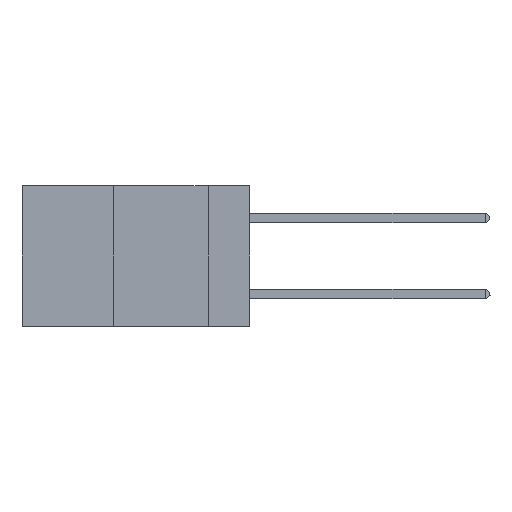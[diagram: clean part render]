
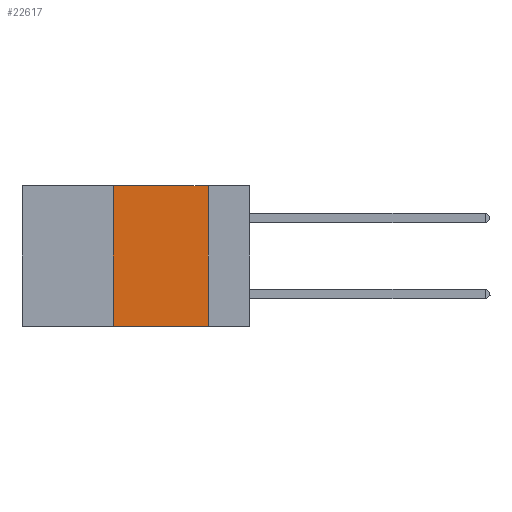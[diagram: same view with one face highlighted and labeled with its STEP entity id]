
A CAD part, left-side view. The second image highlights one B-rep face of the part: STEP entity #22617.
In plain terms, the highlighted planar face has unit normal (-1, 0, 0).
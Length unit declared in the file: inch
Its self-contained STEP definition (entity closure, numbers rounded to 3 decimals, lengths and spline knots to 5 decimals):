
#1865 = VERTEX_POINT ( 'NONE', #22115 ) ;
#2059 = CARTESIAN_POINT ( 'NONE',  ( 0., 0.11, 0. ) ) ;
#3013 = EDGE_LOOP ( 'NONE', ( #31427, #17094, #28552, #44495 ) ) ;
#3513 = DIRECTION ( 'NONE',  ( 0., 0., -1. ) ) ;
#3984 = CARTESIAN_POINT ( 'NONE',  ( 0., 0.11, 0. ) ) ;
#5112 = LINE ( 'NONE', #32090, #32329 ) ;
#7282 = DIRECTION ( 'NONE',  ( 0., -1., 0. ) ) ;
#7284 = CARTESIAN_POINT ( 'NONE',  ( 0., 0.6, 0. ) ) ;
#9518 = DIRECTION ( 'NONE',  ( 0., -1., 0. ) ) ;
#12068 = LINE ( 'NONE', #3984, #15471 ) ;
#12148 = EDGE_CURVE ( 'NONE', #43006, #32721, #12068, .T. ) ;
#15296 = FACE_OUTER_BOUND ( 'NONE', #3013, .T. ) ;
#15455 = CARTESIAN_POINT ( 'NONE',  ( 0., 0.11, -0.37 ) ) ;
#15471 = VECTOR ( 'NONE', #3513, 39.37008 ) ;
#17094 = ORIENTED_EDGE ( 'NONE', *, *, #31562, .F. ) ;
#21498 = PLANE ( 'NONE',  #27385 ) ;
#22115 = CARTESIAN_POINT ( 'NONE',  ( 0., 0.36, 0. ) ) ;
#22410 = CARTESIAN_POINT ( 'NONE',  ( 0., 0.36, -0.37 ) ) ;
#22533 = EDGE_CURVE ( 'NONE', #39396, #1865, #28602, .T. ) ;
#22617 = ADVANCED_FACE ( 'NONE', ( #15296 ), #21498, .F. ) ;
#24997 = EDGE_CURVE ( 'NONE', #39396, #32721, #5112, .T. ) ;
#27385 = AXIS2_PLACEMENT_3D ( 'NONE', #7284, #32092, #28964 ) ;
#28552 = ORIENTED_EDGE ( 'NONE', *, *, #22533, .F. ) ;
#28602 = LINE ( 'NONE', #39047, #42508 ) ;
#28964 = DIRECTION ( 'NONE',  ( 0., 0., -1. ) ) ;
#29127 = VECTOR ( 'NONE', #9518, 39.37008 ) ;
#31427 = ORIENTED_EDGE ( 'NONE', *, *, #12148, .F. ) ;
#31562 = EDGE_CURVE ( 'NONE', #1865, #43006, #38551, .T. ) ;
#32090 = CARTESIAN_POINT ( 'NONE',  ( 0., 0.6, -0.37 ) ) ;
#32092 = DIRECTION ( 'NONE',  ( 1., 0., 0. ) ) ;
#32329 = VECTOR ( 'NONE', #7282, 39.37008 ) ;
#32721 = VERTEX_POINT ( 'NONE', #15455 ) ;
#35493 = DIRECTION ( 'NONE',  ( 0., 0., 1. ) ) ;
#38551 = LINE ( 'NONE', #41612, #29127 ) ;
#39047 = CARTESIAN_POINT ( 'NONE',  ( 0., 0.36, 0. ) ) ;
#39396 = VERTEX_POINT ( 'NONE', #22410 ) ;
#41612 = CARTESIAN_POINT ( 'NONE',  ( 0., 0.6, 0. ) ) ;
#42508 = VECTOR ( 'NONE', #35493, 39.37008 ) ;
#43006 = VERTEX_POINT ( 'NONE', #2059 ) ;
#44495 = ORIENTED_EDGE ( 'NONE', *, *, #24997, .T. ) ;
